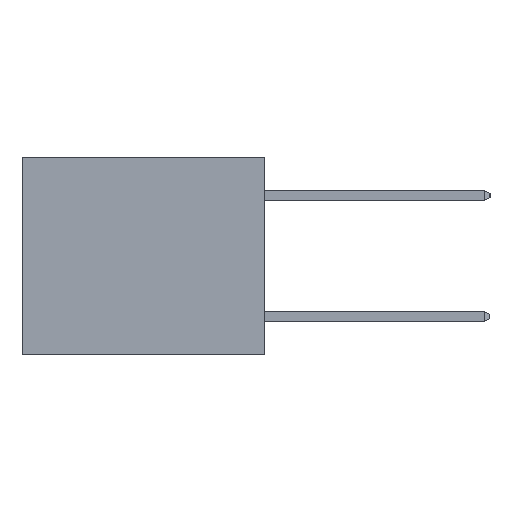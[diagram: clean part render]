
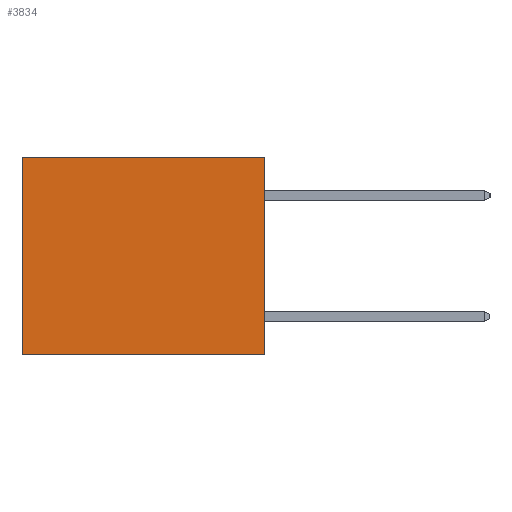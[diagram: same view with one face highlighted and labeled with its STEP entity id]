
A CAD part, left-side view. The second image highlights one B-rep face of the part: STEP entity #3834.
In plain terms, the highlighted planar face has unit normal (-1, 0, 0).
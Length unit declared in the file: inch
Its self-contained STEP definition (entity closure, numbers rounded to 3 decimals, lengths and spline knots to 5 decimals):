
#89 = ORIENTED_EDGE ( 'NONE', *, *, #4237, .F. ) ;
#1445 = AXIS2_PLACEMENT_3D ( 'NONE', #12437, #3176, #11296 ) ;
#1926 = DIRECTION ( 'NONE',  ( 0., 1., 0. ) ) ;
#2095 = VECTOR ( 'NONE', #10956, 39.37008 ) ;
#2996 = VERTEX_POINT ( 'NONE', #14518 ) ;
#3176 = DIRECTION ( 'NONE',  ( 1., 0., 0. ) ) ;
#3834 = ADVANCED_FACE ( 'NONE', ( #16367 ), #12499, .F. ) ;
#4237 = EDGE_CURVE ( 'NONE', #4490, #7446, #14030, .T. ) ;
#4490 = VERTEX_POINT ( 'NONE', #11834 ) ;
#4637 = ORIENTED_EDGE ( 'NONE', *, *, #10318, .T. ) ;
#5819 = VERTEX_POINT ( 'NONE', #9180 ) ;
#6132 = CARTESIAN_POINT ( 'NONE',  ( 0.3165, 0., -0.49 ) ) ;
#6829 = VECTOR ( 'NONE', #1926, 39.37008 ) ;
#7082 = ORIENTED_EDGE ( 'NONE', *, *, #17282, .T. ) ;
#7109 = CARTESIAN_POINT ( 'NONE',  ( 0.3165, 0., -0.49 ) ) ;
#7446 = VERTEX_POINT ( 'NONE', #10590 ) ;
#8121 = LINE ( 'NONE', #6132, #6829 ) ;
#8447 = EDGE_LOOP ( 'NONE', ( #4637, #16599, #89, #7082 ) ) ;
#9180 = CARTESIAN_POINT ( 'NONE',  ( 0.3165, 0.6, 0. ) ) ;
#10318 = EDGE_CURVE ( 'NONE', #5819, #2996, #17391, .T. ) ;
#10590 = CARTESIAN_POINT ( 'NONE',  ( 0.3165, 0., -0.49 ) ) ;
#10956 = DIRECTION ( 'NONE',  ( 0., 0., -1. ) ) ;
#11296 = DIRECTION ( 'NONE',  ( 0., 0., -1. ) ) ;
#11379 = DIRECTION ( 'NONE',  ( 0., 1., 0. ) ) ;
#11417 = DIRECTION ( 'NONE',  ( 0., 0., -1. ) ) ;
#11834 = CARTESIAN_POINT ( 'NONE',  ( 0.3165, 0., 0. ) ) ;
#12321 = LINE ( 'NONE', #16788, #17459 ) ;
#12437 = CARTESIAN_POINT ( 'NONE',  ( 0.3165, 0., -0.49 ) ) ;
#12499 = PLANE ( 'NONE',  #1445 ) ;
#14030 = LINE ( 'NONE', #7109, #17212 ) ;
#14518 = CARTESIAN_POINT ( 'NONE',  ( 0.3165, 0.6, -0.49 ) ) ;
#16144 = CARTESIAN_POINT ( 'NONE',  ( 0.3165, 0.6, -0.49 ) ) ;
#16367 = FACE_OUTER_BOUND ( 'NONE', #8447, .T. ) ;
#16599 = ORIENTED_EDGE ( 'NONE', *, *, #17250, .F. ) ;
#16788 = CARTESIAN_POINT ( 'NONE',  ( 0.3165, 0., 0. ) ) ;
#17212 = VECTOR ( 'NONE', #11417, 39.37008 ) ;
#17250 = EDGE_CURVE ( 'NONE', #7446, #2996, #8121, .T. ) ;
#17282 = EDGE_CURVE ( 'NONE', #4490, #5819, #12321, .T. ) ;
#17391 = LINE ( 'NONE', #16144, #2095 ) ;
#17459 = VECTOR ( 'NONE', #11379, 39.37008 ) ;
